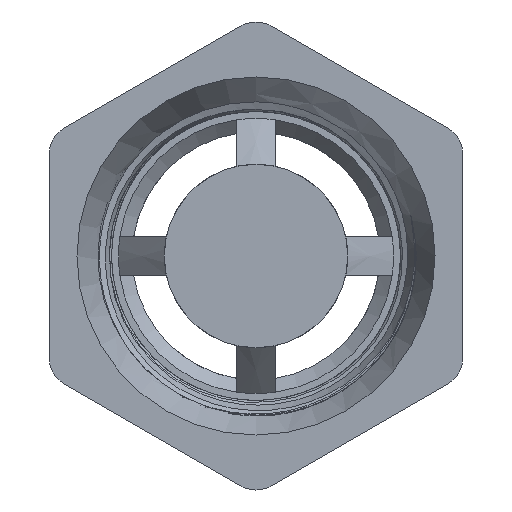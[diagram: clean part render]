
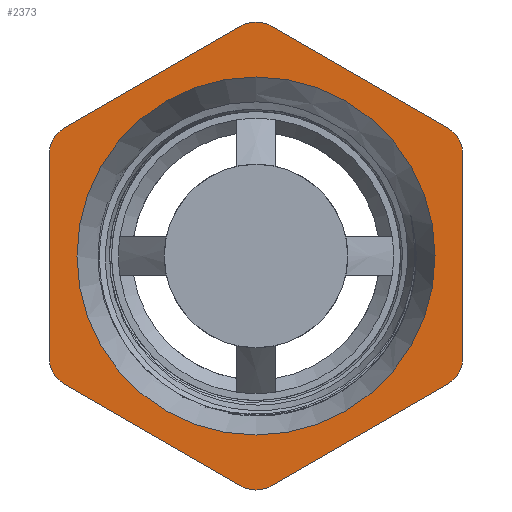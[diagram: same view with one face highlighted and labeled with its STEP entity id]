
A CAD part, front view. The second image highlights one B-rep face of the part: STEP entity #2373.
In plain terms, the highlighted planar face has unit normal (0, -1, 0).
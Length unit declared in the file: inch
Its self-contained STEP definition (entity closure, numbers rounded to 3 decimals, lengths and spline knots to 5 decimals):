
#23=FACE_BOUND('',#363,.T.);
#83=PLANE('',#2621);
#233=FACE_OUTER_BOUND('',#362,.T.);
#362=EDGE_LOOP('',(#2143,#2144,#2145,#2146,#2147,#2148,#2149,#2150,#2151,
#2152,#2153,#2154));
#363=EDGE_LOOP('',(#2155,#2156));
#374=CIRCLE('',#2417,0.46109);
#375=CIRCLE('',#2418,0.46109);
#469=CIRCLE('',#2598,0.07874);
#474=CIRCLE('',#2608,0.07874);
#475=CIRCLE('',#2610,0.07874);
#476=CIRCLE('',#2612,0.07874);
#477=CIRCLE('',#2614,0.07874);
#478=CIRCLE('',#2616,0.07874);
#699=LINE('',#10383,#828);
#715=LINE('',#10505,#844);
#716=LINE('',#10507,#845);
#719=LINE('',#13280,#848);
#720=LINE('',#13281,#849);
#721=LINE('',#13282,#850);
#828=VECTOR('',#3084,0.3937);
#844=VECTOR('',#3188,0.3937);
#845=VECTOR('',#3191,0.3937);
#848=VECTOR('',#3200,0.3937);
#849=VECTOR('',#3201,0.3937);
#850=VECTOR('',#3202,0.3937);
#904=VERTEX_POINT('',#3916);
#905=VERTEX_POINT('',#3917);
#1073=VERTEX_POINT('',#10380);
#1074=VERTEX_POINT('',#10382);
#1081=VERTEX_POINT('',#10465);
#1082=VERTEX_POINT('',#10477);
#1083=VERTEX_POINT('',#10479);
#1084=VERTEX_POINT('',#10483);
#1085=VERTEX_POINT('',#10485);
#1086=VERTEX_POINT('',#10489);
#1087=VERTEX_POINT('',#10491);
#1088=VERTEX_POINT('',#10495);
#1089=VERTEX_POINT('',#10497);
#1090=VERTEX_POINT('',#10501);
#1156=EDGE_CURVE('',#904,#905,#374,.T.);
#1157=EDGE_CURVE('',#905,#904,#375,.T.);
#1410=EDGE_CURVE('',#1074,#1073,#699,.T.);
#1430=EDGE_CURVE('',#1074,#1081,#469,.T.);
#1437=EDGE_CURVE('',#1082,#1083,#474,.T.);
#1440=EDGE_CURVE('',#1084,#1085,#475,.T.);
#1443=EDGE_CURVE('',#1086,#1087,#476,.T.);
#1447=EDGE_CURVE('',#1089,#1088,#477,.T.);
#1448=EDGE_CURVE('',#1090,#1073,#478,.T.);
#1450=EDGE_CURVE('',#1082,#1087,#715,.T.);
#1451=EDGE_CURVE('',#1086,#1081,#716,.T.);
#1458=EDGE_CURVE('',#1090,#1088,#719,.T.);
#1459=EDGE_CURVE('',#1089,#1085,#720,.T.);
#1460=EDGE_CURVE('',#1084,#1083,#721,.T.);
#2143=ORIENTED_EDGE('',*,*,#1437,.F.);
#2144=ORIENTED_EDGE('',*,*,#1450,.T.);
#2145=ORIENTED_EDGE('',*,*,#1443,.F.);
#2146=ORIENTED_EDGE('',*,*,#1451,.T.);
#2147=ORIENTED_EDGE('',*,*,#1430,.F.);
#2148=ORIENTED_EDGE('',*,*,#1410,.T.);
#2149=ORIENTED_EDGE('',*,*,#1448,.F.);
#2150=ORIENTED_EDGE('',*,*,#1458,.T.);
#2151=ORIENTED_EDGE('',*,*,#1447,.F.);
#2152=ORIENTED_EDGE('',*,*,#1459,.T.);
#2153=ORIENTED_EDGE('',*,*,#1440,.F.);
#2154=ORIENTED_EDGE('',*,*,#1460,.T.);
#2155=ORIENTED_EDGE('',*,*,#1156,.T.);
#2156=ORIENTED_EDGE('',*,*,#1157,.T.);
#2373=ADVANCED_FACE('',(#233,#23),#83,.T.);
#2417=AXIS2_PLACEMENT_3D('',#3918,#2677,#2678);
#2418=AXIS2_PLACEMENT_3D('',#3919,#2679,#2680);
#2598=AXIS2_PLACEMENT_3D('',#10466,#3138,#3139);
#2608=AXIS2_PLACEMENT_3D('',#10480,#3160,#3161);
#2610=AXIS2_PLACEMENT_3D('',#10486,#3166,#3167);
#2612=AXIS2_PLACEMENT_3D('',#10492,#3172,#3173);
#2614=AXIS2_PLACEMENT_3D('',#10499,#3179,#3180);
#2616=AXIS2_PLACEMENT_3D('',#10502,#3183,#3184);
#2621=AXIS2_PLACEMENT_3D('',#13279,#3198,#3199);
#2677=DIRECTION('center_axis',(0.,1.,0.));
#2678=DIRECTION('ref_axis',(0.,0.,-1.));
#2679=DIRECTION('center_axis',(0.,1.,0.));
#2680=DIRECTION('ref_axis',(0.,0.,-1.));
#3084=DIRECTION('',(0.,0.,1.));
#3138=DIRECTION('center_axis',(0.,1.,0.));
#3139=DIRECTION('ref_axis',(0.866,0.,-0.5));
#3160=DIRECTION('center_axis',(0.,1.,0.));
#3161=DIRECTION('ref_axis',(-0.866,0.,-0.5));
#3166=DIRECTION('center_axis',(0.,1.,0.));
#3167=DIRECTION('ref_axis',(-0.866,0.,0.5));
#3172=DIRECTION('center_axis',(0.,1.,0.));
#3173=DIRECTION('ref_axis',(0.,0.,-1.));
#3179=DIRECTION('center_axis',(0.,1.,0.));
#3180=DIRECTION('ref_axis',(0.,0.,1.));
#3183=DIRECTION('center_axis',(0.,1.,0.));
#3184=DIRECTION('ref_axis',(0.866,0.,0.5));
#3188=DIRECTION('',(0.866,0.,-0.5));
#3191=DIRECTION('',(0.866,0.,0.5));
#3198=DIRECTION('center_axis',(0.,-1.,0.));
#3199=DIRECTION('ref_axis',(0.,0.,-1.));
#3200=DIRECTION('',(-0.866,0.,0.5));
#3201=DIRECTION('',(-0.866,0.,-0.5));
#3202=DIRECTION('',(0.,0.,-1.));
#3916=CARTESIAN_POINT('',(0.,-1.,-0.46109));
#3917=CARTESIAN_POINT('',(0.,-1.,0.46109));
#3918=CARTESIAN_POINT('Origin',(0.,-1.,0.));
#3919=CARTESIAN_POINT('Origin',(0.,-1.,0.));
#10380=CARTESIAN_POINT('',(0.53242,-1.,0.26193));
#10382=CARTESIAN_POINT('',(0.53242,-1.,-0.26193));
#10383=CARTESIAN_POINT('',(0.53242,-1.,-0.30739));
#10465=CARTESIAN_POINT('',(0.49305,-1.,-0.33012));
#10466=CARTESIAN_POINT('Origin',(0.45368,-1.,-0.26193));
#10477=CARTESIAN_POINT('',(-0.49305,-1.,-0.33012));
#10479=CARTESIAN_POINT('',(-0.53242,-1.,-0.26193));
#10480=CARTESIAN_POINT('Origin',(-0.45368,-1.,-0.26193));
#10483=CARTESIAN_POINT('',(-0.53242,-1.,0.26193));
#10485=CARTESIAN_POINT('',(-0.49305,-1.,0.33012));
#10486=CARTESIAN_POINT('Origin',(-0.45368,-1.,0.26193));
#10489=CARTESIAN_POINT('',(0.03937,-1.,-0.59206));
#10491=CARTESIAN_POINT('',(-0.03937,-1.,-0.59206));
#10492=CARTESIAN_POINT('Origin',(0.,-1.,-0.52387));
#10495=CARTESIAN_POINT('',(0.03937,-1.,0.59206));
#10497=CARTESIAN_POINT('',(-0.03937,-1.,0.59206));
#10499=CARTESIAN_POINT('Origin',(0.,-1.,0.52387));
#10501=CARTESIAN_POINT('',(0.49305,-1.,0.33012));
#10502=CARTESIAN_POINT('Origin',(0.45368,-1.,0.26193));
#10505=CARTESIAN_POINT('',(-0.53242,-1.,-0.30739));
#10507=CARTESIAN_POINT('',(0.,-1.,-0.61479));
#13279=CARTESIAN_POINT('Origin',(0.,-1.,0.));
#13280=CARTESIAN_POINT('',(0.53242,-1.,0.30739));
#13281=CARTESIAN_POINT('',(0.,-1.,0.61479));
#13282=CARTESIAN_POINT('',(-0.53242,-1.,0.30739));
